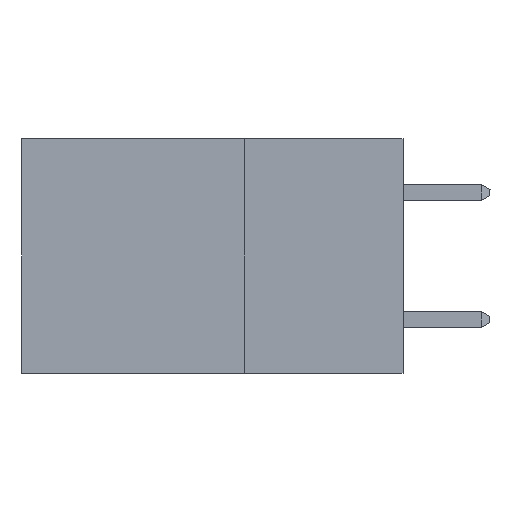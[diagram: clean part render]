
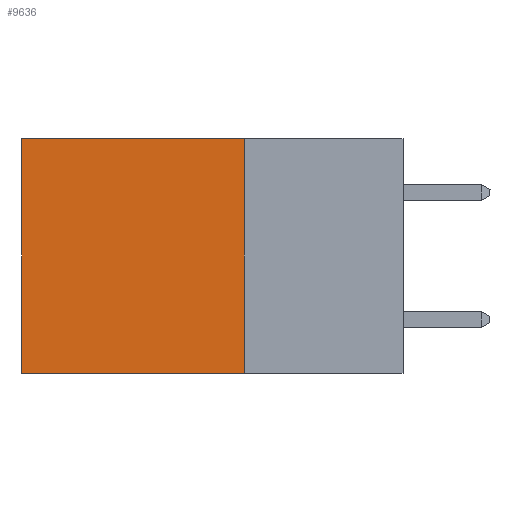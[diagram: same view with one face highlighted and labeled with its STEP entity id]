
A CAD part, left-side view. The second image highlights one B-rep face of the part: STEP entity #9636.
In plain terms, the highlighted planar face has unit normal (-1, 0, 0).
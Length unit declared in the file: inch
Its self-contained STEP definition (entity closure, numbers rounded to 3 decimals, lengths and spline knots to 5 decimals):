
#13 = EDGE_CURVE ( 'NONE', #8063, #12640, #9102, .T. ) ;
#93 = EDGE_CURVE ( 'NONE', #12640, #3846, #7954, .T. ) ;
#751 = CARTESIAN_POINT ( 'NONE',  ( 0.2875, 0.6, 0. ) ) ;
#963 = CARTESIAN_POINT ( 'NONE',  ( 0.2875, 0.25, 0. ) ) ;
#1339 = CARTESIAN_POINT ( 'NONE',  ( 0.2875, 0.25, 0. ) ) ;
#2645 = DIRECTION ( 'NONE',  ( 1., 0., 0. ) ) ;
#2805 = ORIENTED_EDGE ( 'NONE', *, *, #12946, .F. ) ;
#3162 = LINE ( 'NONE', #14872, #12561 ) ;
#3315 = DIRECTION ( 'NONE',  ( 0., 0., -1. ) ) ;
#3552 = VERTEX_POINT ( 'NONE', #6268 ) ;
#3666 = VECTOR ( 'NONE', #7405, 39.37008 ) ;
#3846 = VERTEX_POINT ( 'NONE', #14017 ) ;
#4687 = VECTOR ( 'NONE', #3315, 39.37008 ) ;
#5150 = DIRECTION ( 'NONE',  ( 0., 1., 0. ) ) ;
#5358 = CARTESIAN_POINT ( 'NONE',  ( 0.2875, 0.25, 0. ) ) ;
#5609 = AXIS2_PLACEMENT_3D ( 'NONE', #1339, #2645, #11264 ) ;
#5680 = ORIENTED_EDGE ( 'NONE', *, *, #13, .T. ) ;
#5852 = VECTOR ( 'NONE', #5150, 39.37008 ) ;
#6268 = CARTESIAN_POINT ( 'NONE',  ( 0.2875, 0.25, -0.37 ) ) ;
#6806 = FACE_OUTER_BOUND ( 'NONE', #13673, .T. ) ;
#6909 = ORIENTED_EDGE ( 'NONE', *, *, #14452, .F. ) ;
#7405 = DIRECTION ( 'NONE',  ( 0., 0., -1. ) ) ;
#7954 = LINE ( 'NONE', #9573, #4687 ) ;
#8063 = VERTEX_POINT ( 'NONE', #963 ) ;
#8870 = PLANE ( 'NONE',  #5609 ) ;
#9102 = LINE ( 'NONE', #5358, #5852 ) ;
#9573 = CARTESIAN_POINT ( 'NONE',  ( 0.2875, 0.6, 0. ) ) ;
#9636 = ADVANCED_FACE ( 'NONE', ( #6806 ), #8870, .F. ) ;
#10975 = ORIENTED_EDGE ( 'NONE', *, *, #93, .T. ) ;
#11264 = DIRECTION ( 'NONE',  ( 0., 0., -1. ) ) ;
#12195 = CARTESIAN_POINT ( 'NONE',  ( 0.2875, 0.25, 0. ) ) ;
#12561 = VECTOR ( 'NONE', #13695, 39.37008 ) ;
#12640 = VERTEX_POINT ( 'NONE', #751 ) ;
#12946 = EDGE_CURVE ( 'NONE', #3552, #3846, #3162, .T. ) ;
#13406 = LINE ( 'NONE', #12195, #3666 ) ;
#13673 = EDGE_LOOP ( 'NONE', ( #10975, #2805, #6909, #5680 ) ) ;
#13695 = DIRECTION ( 'NONE',  ( 0., 1., 0. ) ) ;
#14017 = CARTESIAN_POINT ( 'NONE',  ( 0.2875, 0.6, -0.37 ) ) ;
#14452 = EDGE_CURVE ( 'NONE', #8063, #3552, #13406, .T. ) ;
#14872 = CARTESIAN_POINT ( 'NONE',  ( 0.2875, 0.25, -0.37 ) ) ;
